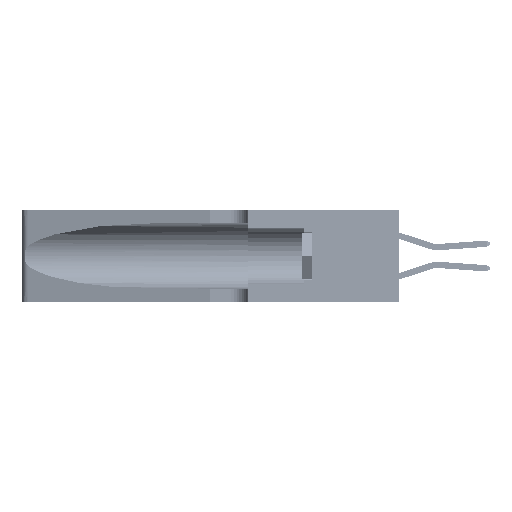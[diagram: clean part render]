
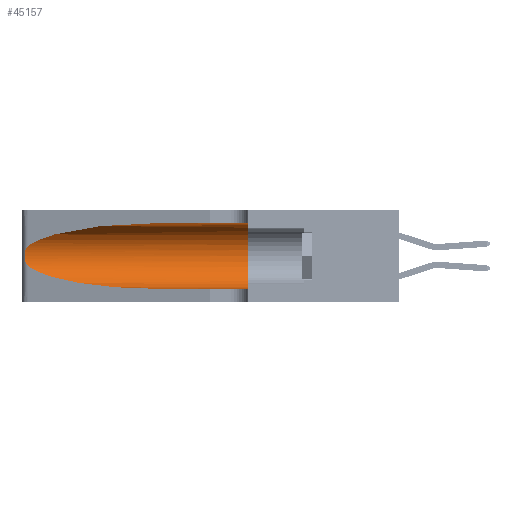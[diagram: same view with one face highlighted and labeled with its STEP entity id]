
A CAD part, left-side view. The second image highlights one B-rep face of the part: STEP entity #45157.
In plain terms, the highlighted cylindrical face has radius 3.308 mm (diameter 6.617 mm), a partial arc.
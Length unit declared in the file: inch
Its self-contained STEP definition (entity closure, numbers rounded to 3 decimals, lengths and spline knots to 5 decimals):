
#707 = CARTESIAN_POINT ( 'NONE',  ( 0.18966, 0.96281, 0.05475 ) ) ;
#726 = CARTESIAN_POINT ( 'NONE',  ( 0.1305, 0.72297, 0.05475 ) ) ;
#945 = AXIS2_PLACEMENT_3D ( 'NONE', #29818, #37633, #14428 ) ;
#1757 = VECTOR ( 'NONE', #29864, 39.37008 ) ;
#2969 = LINE ( 'NONE', #6687, #1757 ) ;
#3252 = CARTESIAN_POINT ( 'NONE',  ( 0.26075, 1.23896, 0.178 ) ) ;
#3707 = CARTESIAN_POINT ( 'NONE',  ( 0.25487, 1.22718, 0.14631 ) ) ;
#4115 = EDGE_LOOP ( 'NONE', ( #27940, #24231, #9660, #6369, #15740, #33477 ) ) ;
#4290 = VECTOR ( 'NONE', #46684, 39.37008 ) ;
#4455 = CARTESIAN_POINT ( 'NONE',  ( 0.1305, 0.35, 0.05475 ) ) ;
#6369 = ORIENTED_EDGE ( 'NONE', *, *, #27893, .T. ) ;
#6687 = CARTESIAN_POINT ( 'NONE',  ( 0.1305, 1.61858, 0.05475 ) ) ;
#7139 = CARTESIAN_POINT ( 'NONE',  ( 0.25856, 1.23593, 0.16098 ) ) ;
#7939 =( BOUNDED_CURVE ( )  B_SPLINE_CURVE ( 3, ( #13381, #9323, #21114, #48264 ),
 .UNSPECIFIED., .F., .T. ) 
 B_SPLINE_CURVE_WITH_KNOTS ( ( 4, 4 ),
 ( 1.5708, 2.84003 ),
 .UNSPECIFIED. ) 
 CURVE ( )  GEOMETRIC_REPRESENTATION_ITEM ( )  RATIONAL_B_SPLINE_CURVE ( ( 1., 0.87, 0.87, 1. ) ) 
 REPRESENTATION_ITEM ( '' )  );
#9323 = CARTESIAN_POINT ( 'NONE',  ( 0.18966, 0.96281, 0.31525 ) ) ;
#9660 = ORIENTED_EDGE ( 'NONE', *, *, #13024, .T. ) ;
#11059 = CARTESIAN_POINT ( 'NONE',  ( 0.25639, 1.23186, 0.15144 ) ) ;
#12073 = VERTEX_POINT ( 'NONE', #49399 ) ;
#12376 = CIRCLE ( 'NONE', #15916, 0.13025 ) ;
#12420 = CARTESIAN_POINT ( 'NONE',  ( 0.25487, 1.22718, 0.14631 ) ) ;
#13024 = EDGE_CURVE ( 'NONE', #26828, #28172, #38677, .T. ) ;
#13381 = CARTESIAN_POINT ( 'NONE',  ( 0.1305, 0.72297, 0.31525 ) ) ;
#14428 = DIRECTION ( 'NONE',  ( 0., 0., -1. ) ) ;
#14762 = CARTESIAN_POINT ( 'NONE',  ( 0.25487, 1.22718, 0.22369 ) ) ;
#14937 = CARTESIAN_POINT ( 'NONE',  ( 0.25487, 1.22718, 0.14631 ) ) ;
#15740 = ORIENTED_EDGE ( 'NONE', *, *, #47450, .F. ) ;
#15916 = AXIS2_PLACEMENT_3D ( 'NONE', #42841, #19627, #46770 ) ;
#16447 = CARTESIAN_POINT ( 'NONE',  ( 0.1305, 0.72297, 0.31525 ) ) ;
#18648 = CARTESIAN_POINT ( 'NONE',  ( 0.25639, 1.23184, 0.21858 ) ) ;
#19627 = DIRECTION ( 'NONE',  ( 0., 1., 0. ) ) ;
#21114 = CARTESIAN_POINT ( 'NONE',  ( 0.2373, 1.15595, 0.28018 ) ) ;
#22525 = CARTESIAN_POINT ( 'NONE',  ( 0.25854, 1.2359, 0.20912 ) ) ;
#22953 = CARTESIAN_POINT ( 'NONE',  ( 0.1305, 0.35, 0.31525 ) ) ;
#23414 = CARTESIAN_POINT ( 'NONE',  ( 0.1305, 1.61858, 0.31525 ) ) ;
#24231 = ORIENTED_EDGE ( 'NONE', *, *, #42292, .T. ) ;
#26428 = CARTESIAN_POINT ( 'NONE',  ( 0.26075, 1.23896, 0.19203 ) ) ;
#26828 = VERTEX_POINT ( 'NONE', #3707 ) ;
#27893 = EDGE_CURVE ( 'NONE', #28172, #28166, #2969, .T. ) ;
#27940 = ORIENTED_EDGE ( 'NONE', *, *, #41102, .T. ) ;
#28166 = VERTEX_POINT ( 'NONE', #4455 ) ;
#28172 = VERTEX_POINT ( 'NONE', #726 ) ;
#29817 = VERTEX_POINT ( 'NONE', #22953 ) ;
#29818 = CARTESIAN_POINT ( 'NONE',  ( 0.1305, 1.61858, 0.185 ) ) ;
#29864 = DIRECTION ( 'NONE',  ( 0., -1., 0. ) ) ;
#30340 = CARTESIAN_POINT ( 'NONE',  ( 0.26017, 1.23833, 0.17102 ) ) ;
#30430 = FACE_OUTER_BOUND ( 'NONE', #4115, .T. ) ;
#32864 = EDGE_CURVE ( 'NONE', #37451, #29817, #46050, .T. ) ;
#33477 = ORIENTED_EDGE ( 'NONE', *, *, #32864, .F. ) ;
#34241 = CARTESIAN_POINT ( 'NONE',  ( 0.25789, 1.23486, 0.15765 ) ) ;
#37451 = VERTEX_POINT ( 'NONE', #16447 ) ;
#37633 = DIRECTION ( 'NONE',  ( 0., -1., 0. ) ) ;
#38132 = CARTESIAN_POINT ( 'NONE',  ( 0.25555, 1.22993, 0.14849 ) ) ;
#38677 =( BOUNDED_CURVE ( )  B_SPLINE_CURVE ( 3, ( #12420, #39330, #707, #39501 ),
 .UNSPECIFIED., .F., .F. ) 
 B_SPLINE_CURVE_WITH_KNOTS ( ( 4, 4 ),
 ( 3.44316, 4.71239 ),
 .UNSPECIFIED. ) 
 CURVE ( )  GEOMETRIC_REPRESENTATION_ITEM ( )  RATIONAL_B_SPLINE_CURVE ( ( 1., 0.87, 0.87, 1. ) ) 
 REPRESENTATION_ITEM ( '' )  );
#39330 = CARTESIAN_POINT ( 'NONE',  ( 0.2373, 1.15595, 0.08982 ) ) ;
#39501 = CARTESIAN_POINT ( 'NONE',  ( 0.1305, 0.72297, 0.05475 ) ) ;
#41102 = EDGE_CURVE ( 'NONE', #37451, #12073, #7939, .T. ) ;
#41866 = CARTESIAN_POINT ( 'NONE',  ( 0.25555, 1.22994, 0.2215 ) ) ;
#42292 = EDGE_CURVE ( 'NONE', #12073, #26828, #49223, .T. ) ;
#42841 = CARTESIAN_POINT ( 'NONE',  ( 0.1305, 0.35, 0.185 ) ) ;
#45157 = ADVANCED_FACE ( 'NONE', ( #30430 ), #48630, .F. ) ;
#45774 = CARTESIAN_POINT ( 'NONE',  ( 0.25787, 1.23484, 0.2124 ) ) ;
#46050 = LINE ( 'NONE', #23414, #4290 ) ;
#46684 = DIRECTION ( 'NONE',  ( 0., -1., 0. ) ) ;
#46770 = DIRECTION ( 'NONE',  ( 0., 0., 1. ) ) ;
#47450 = EDGE_CURVE ( 'NONE', #29817, #28166, #12376, .T. ) ;
#48264 = CARTESIAN_POINT ( 'NONE',  ( 0.25487, 1.22718, 0.22369 ) ) ;
#48630 = CYLINDRICAL_SURFACE ( 'NONE', #945, 0.13025 ) ;
#49223 = B_SPLINE_CURVE_WITH_KNOTS ( 'NONE', 3,
 ( #14762, #41866, #18648, #45774, #22525, #49662, #26428, #3252, #30340, #7139, #34241, #11059, #38132, #14937 ),
 .UNSPECIFIED., .F., .F.,
 ( 4, 2, 2, 2, 2, 2, 4 ),
 ( 0., 0.00027, 0.00053, 0.00107, 0.0016, 0.00187, 0.00214 ),
 .UNSPECIFIED. ) ;
#49399 = CARTESIAN_POINT ( 'NONE',  ( 0.25487, 1.22718, 0.22369 ) ) ;
#49662 = CARTESIAN_POINT ( 'NONE',  ( 0.26018, 1.23835, 0.19895 ) ) ;
